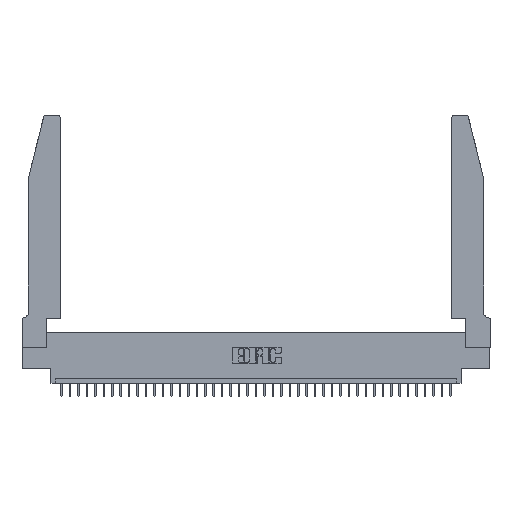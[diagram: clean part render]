
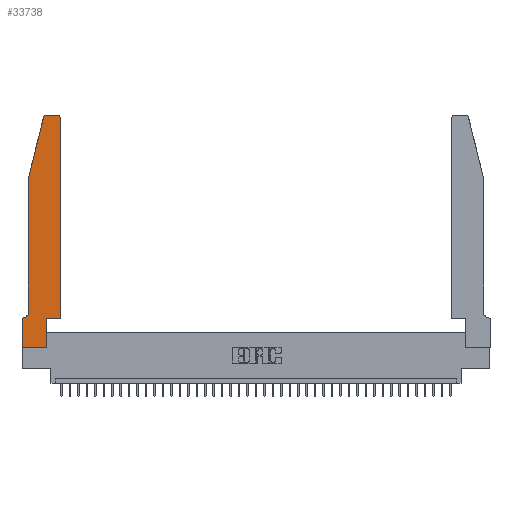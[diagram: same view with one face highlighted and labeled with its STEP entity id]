
A CAD part, top view. The second image highlights one B-rep face of the part: STEP entity #33738.
In plain terms, the highlighted planar face has unit normal (0, 0, 1).
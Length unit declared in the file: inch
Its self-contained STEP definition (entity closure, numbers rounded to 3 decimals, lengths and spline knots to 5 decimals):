
#102 = EDGE_LOOP ( 'NONE', ( #7127, #23148, #20854, #37068, #24875, #11547, #22182, #136, #157, #1575, #10107, #6028 ) ) ;
#112 = VECTOR ( 'NONE', #29565, 39.37008 ) ;
#136 = ORIENTED_EDGE ( 'NONE', *, *, #22071, .T. ) ;
#157 = ORIENTED_EDGE ( 'NONE', *, *, #35252, .T. ) ;
#498 = CARTESIAN_POINT ( 'NONE',  ( 0.4505, 0.35, 0.37 ) ) ;
#798 = DIRECTION ( 'NONE',  ( 0., 0., 1. ) ) ;
#996 = DIRECTION ( 'NONE',  ( 0., -1., 0. ) ) ;
#1475 = CARTESIAN_POINT ( 'NONE',  ( 0.4505, 0.35, 0.37 ) ) ;
#1575 = ORIENTED_EDGE ( 'NONE', *, *, #23127, .T. ) ;
#2193 = LINE ( 'NONE', #2519, #36666 ) ;
#2519 = CARTESIAN_POINT ( 'NONE',  ( 0., 0., 0.37 ) ) ;
#3074 = VERTEX_POINT ( 'NONE', #9425 ) ;
#3770 = DIRECTION ( 'NONE',  ( 1., 0., 0. ) ) ;
#4141 = LINE ( 'NONE', #17267, #34801 ) ;
#4238 = LINE ( 'NONE', #27762, #37239 ) ;
#4706 = DIRECTION ( 'NONE',  ( 0., 1., 0. ) ) ;
#4976 = EDGE_CURVE ( 'NONE', #16089, #27476, #5456, .T. ) ;
#5040 = CIRCLE ( 'NONE', #19872, 0.03 ) ;
#5456 = LINE ( 'NONE', #22259, #11173 ) ;
#6028 = ORIENTED_EDGE ( 'NONE', *, *, #12587, .T. ) ;
#6108 = VERTEX_POINT ( 'NONE', #24623 ) ;
#6403 = DIRECTION ( 'NONE',  ( 1., 0., 0. ) ) ;
#6560 = CARTESIAN_POINT ( 'NONE',  ( 0.2865, 0.35, 0.37 ) ) ;
#7127 = ORIENTED_EDGE ( 'NONE', *, *, #32337, .T. ) ;
#7409 = CARTESIAN_POINT ( 'NONE',  ( 0.284, 2.75, 0.37 ) ) ;
#7511 = EDGE_CURVE ( 'NONE', #12049, #38438, #4238, .T. ) ;
#7680 = CARTESIAN_POINT ( 'NONE',  ( 0.25487, 2.72718, 0.37 ) ) ;
#8368 = DIRECTION ( 'NONE',  ( 0., 0., 1. ) ) ;
#8395 = CARTESIAN_POINT ( 'NONE',  ( 0.0755, 2., 0.37 ) ) ;
#8406 = CARTESIAN_POINT ( 'NONE',  ( 0.2605, 2.75, 0.37 ) ) ;
#8442 = CARTESIAN_POINT ( 'NONE',  ( 0.284, 2.72, 0.37 ) ) ;
#9425 = CARTESIAN_POINT ( 'NONE',  ( 0.2865, 0., 0.37 ) ) ;
#10013 = EDGE_CURVE ( 'NONE', #28763, #16089, #11207, .T. ) ;
#10107 = ORIENTED_EDGE ( 'NONE', *, *, #38923, .T. ) ;
#11173 = VECTOR ( 'NONE', #996, 39.37008 ) ;
#11207 = LINE ( 'NONE', #8395, #37519 ) ;
#11547 = ORIENTED_EDGE ( 'NONE', *, *, #7511, .T. ) ;
#11744 = CIRCLE ( 'NONE', #34798, 0.03 ) ;
#12049 = VERTEX_POINT ( 'NONE', #26522 ) ;
#12381 = DIRECTION ( 'NONE',  ( -1., 0., 0. ) ) ;
#12551 = VERTEX_POINT ( 'NONE', #34819 ) ;
#12587 = EDGE_CURVE ( 'NONE', #6108, #12551, #5040, .T. ) ;
#12956 = CARTESIAN_POINT ( 'NONE',  ( 0.0755, 0.42, 0.37 ) ) ;
#14036 = CARTESIAN_POINT ( 'NONE',  ( 0., 0., 0.37 ) ) ;
#14429 = DIRECTION ( 'NONE',  ( 0., -1., 0. ) ) ;
#14444 = DIRECTION ( 'NONE',  ( -1., 0., 0. ) ) ;
#15398 = VECTOR ( 'NONE', #6403, 39.37008 ) ;
#16089 = VERTEX_POINT ( 'NONE', #31463 ) ;
#17233 = FACE_OUTER_BOUND ( 'NONE', #102, .T. ) ;
#17267 = CARTESIAN_POINT ( 'NONE',  ( 0.2865, 0.35, 0.37 ) ) ;
#17377 = LINE ( 'NONE', #498, #15398 ) ;
#17450 = VECTOR ( 'NONE', #4706, 39.37008 ) ;
#17582 = VERTEX_POINT ( 'NONE', #6560 ) ;
#18376 = LINE ( 'NONE', #1475, #17450 ) ;
#18467 = CARTESIAN_POINT ( 'NONE',  ( 0.4505, 0.35, 0.37 ) ) ;
#18914 = CARTESIAN_POINT ( 'NONE',  ( 0., 0., 0.37 ) ) ;
#19661 = VERTEX_POINT ( 'NONE', #18914 ) ;
#19872 = AXIS2_PLACEMENT_3D ( 'NONE', #37365, #798, #3770 ) ;
#20587 = EDGE_CURVE ( 'NONE', #38438, #19661, #2193, .T. ) ;
#20833 = DIRECTION ( 'NONE',  ( 1., 0., 0. ) ) ;
#20854 = ORIENTED_EDGE ( 'NONE', *, *, #10013, .T. ) ;
#20953 = CARTESIAN_POINT ( 'NONE',  ( 0., 0.35, 0.37 ) ) ;
#21089 = VECTOR ( 'NONE', #14444, 39.37008 ) ;
#22071 = EDGE_CURVE ( 'NONE', #19661, #3074, #38958, .T. ) ;
#22182 = ORIENTED_EDGE ( 'NONE', *, *, #20587, .T. ) ;
#22259 = CARTESIAN_POINT ( 'NONE',  ( 0.0755, 2., 0.37 ) ) ;
#23127 = EDGE_CURVE ( 'NONE', #17582, #32938, #17377, .T. ) ;
#23148 = ORIENTED_EDGE ( 'NONE', *, *, #29875, .T. ) ;
#23582 = CARTESIAN_POINT ( 'NONE',  ( 0.0055, 0.42, 0.37 ) ) ;
#23685 = DIRECTION ( 'NONE',  ( 1., 0., 0. ) ) ;
#24297 = AXIS2_PLACEMENT_3D ( 'NONE', #20953, #8368, #20833 ) ;
#24623 = CARTESIAN_POINT ( 'NONE',  ( 0.4505, 2.72, 0.37 ) ) ;
#24875 = ORIENTED_EDGE ( 'NONE', *, *, #28854, .T. ) ;
#26522 = CARTESIAN_POINT ( 'NONE',  ( 0.0055, 0.35, 0.37 ) ) ;
#26609 = DIRECTION ( 'NONE',  ( 0., 1., 0. ) ) ;
#26990 = DIRECTION ( 'NONE',  ( -0.239, -0.971, 0. ) ) ;
#27476 = VERTEX_POINT ( 'NONE', #12956 ) ;
#27644 = CARTESIAN_POINT ( 'NONE',  ( 0., 0.35, 0.37 ) ) ;
#27762 = CARTESIAN_POINT ( 'NONE',  ( 0.0755, 0.35, 0.37 ) ) ;
#28763 = VERTEX_POINT ( 'NONE', #7680 ) ;
#28854 = EDGE_CURVE ( 'NONE', #27476, #12049, #31264, .T. ) ;
#29514 = DIRECTION ( 'NONE',  ( -1., 0., 0. ) ) ;
#29565 = DIRECTION ( 'NONE',  ( 1., 0., 0. ) ) ;
#29875 = EDGE_CURVE ( 'NONE', #35593, #28763, #11744, .T. ) ;
#30877 = AXIS2_PLACEMENT_3D ( 'NONE', #23582, #32716, #29514 ) ;
#31264 = CIRCLE ( 'NONE', #30877, 0.07 ) ;
#31463 = CARTESIAN_POINT ( 'NONE',  ( 0.0755, 2., 0.37 ) ) ;
#32337 = EDGE_CURVE ( 'NONE', #12551, #35593, #35049, .T. ) ;
#32716 = DIRECTION ( 'NONE',  ( 0., 0., -1. ) ) ;
#32727 = PLANE ( 'NONE',  #24297 ) ;
#32938 = VERTEX_POINT ( 'NONE', #18467 ) ;
#32944 = DIRECTION ( 'NONE',  ( 0., 0., 1. ) ) ;
#33738 = ADVANCED_FACE ( 'NONE', ( #17233 ), #32727, .T. ) ;
#34798 = AXIS2_PLACEMENT_3D ( 'NONE', #8442, #32944, #23685 ) ;
#34801 = VECTOR ( 'NONE', #26609, 39.37008 ) ;
#34819 = CARTESIAN_POINT ( 'NONE',  ( 0.4205, 2.75, 0.37 ) ) ;
#35049 = LINE ( 'NONE', #8406, #21089 ) ;
#35252 = EDGE_CURVE ( 'NONE', #3074, #17582, #4141, .T. ) ;
#35593 = VERTEX_POINT ( 'NONE', #7409 ) ;
#36666 = VECTOR ( 'NONE', #14429, 39.37008 ) ;
#37068 = ORIENTED_EDGE ( 'NONE', *, *, #4976, .T. ) ;
#37239 = VECTOR ( 'NONE', #12381, 39.37008 ) ;
#37365 = CARTESIAN_POINT ( 'NONE',  ( 0.4205, 2.72, 0.37 ) ) ;
#37519 = VECTOR ( 'NONE', #26990, 39.37008 ) ;
#38438 = VERTEX_POINT ( 'NONE', #27644 ) ;
#38923 = EDGE_CURVE ( 'NONE', #32938, #6108, #18376, .T. ) ;
#38958 = LINE ( 'NONE', #14036, #112 ) ;
